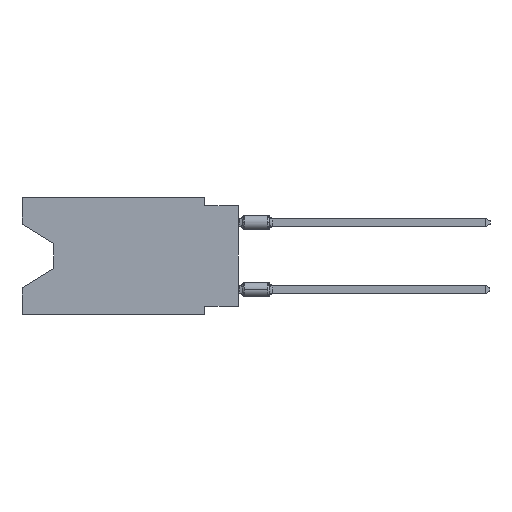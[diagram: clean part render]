
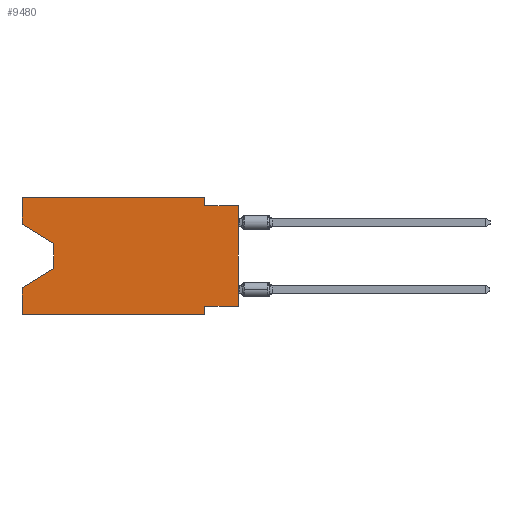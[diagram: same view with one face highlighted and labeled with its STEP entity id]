
A CAD part, left-side view. The second image highlights one B-rep face of the part: STEP entity #9480.
In plain terms, the highlighted planar face has unit normal (-1, 0, 0).
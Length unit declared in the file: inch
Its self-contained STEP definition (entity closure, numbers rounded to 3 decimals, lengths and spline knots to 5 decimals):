
#371 = VECTOR ( 'NONE', #15191, 39.37008 ) ;
#485 = ORIENTED_EDGE ( 'NONE', *, *, #4671, .T. ) ;
#795 = CARTESIAN_POINT ( 'NONE',  ( 0., 0.645, 0. ) ) ;
#812 = VECTOR ( 'NONE', #6958, 39.37008 ) ;
#1088 = DIRECTION ( 'NONE',  ( 0., 0., -1. ) ) ;
#1252 = EDGE_CURVE ( 'NONE', #9907, #4779, #9877, .T. ) ;
#1504 = CARTESIAN_POINT ( 'NONE',  ( 0., 0.1, 0. ) ) ;
#1529 = VECTOR ( 'NONE', #10505, 39.37008 ) ;
#1572 = CARTESIAN_POINT ( 'NONE',  ( 0., 0.55, -0.138 ) ) ;
#1799 = DIRECTION ( 'NONE',  ( 0., 0., -1. ) ) ;
#2082 = CARTESIAN_POINT ( 'NONE',  ( 0., 0.55, -0.138 ) ) ;
#2111 = EDGE_CURVE ( 'NONE', #5982, #10717, #15539, .T. ) ;
#2290 = LINE ( 'NONE', #8749, #15847 ) ;
#2360 = CARTESIAN_POINT ( 'NONE',  ( 0., 0.645, 0. ) ) ;
#2517 = ORIENTED_EDGE ( 'NONE', *, *, #13369, .T. ) ;
#2615 = DIRECTION ( 'NONE',  ( 0., 0.855, -0.519 ) ) ;
#2619 = CARTESIAN_POINT ( 'NONE',  ( 0., 0., -0.325 ) ) ;
#2694 = EDGE_CURVE ( 'NONE', #9907, #5982, #6921, .T. ) ;
#2731 = LINE ( 'NONE', #14497, #12615 ) ;
#3199 = LINE ( 'NONE', #2082, #11906 ) ;
#3293 = CARTESIAN_POINT ( 'NONE',  ( 0., 0., 0. ) ) ;
#4060 = CARTESIAN_POINT ( 'NONE',  ( 0., 0.645, -0.35 ) ) ;
#4140 = VECTOR ( 'NONE', #1088, 39.37008 ) ;
#4315 = CARTESIAN_POINT ( 'NONE',  ( 0., 0.645, 0. ) ) ;
#4490 = CARTESIAN_POINT ( 'NONE',  ( 0., 0., -0.025 ) ) ;
#4505 = LINE ( 'NONE', #10729, #12338 ) ;
#4671 = EDGE_CURVE ( 'NONE', #10297, #6731, #5054, .T. ) ;
#4779 = VERTEX_POINT ( 'NONE', #1572 ) ;
#5054 = LINE ( 'NONE', #6681, #1529 ) ;
#5093 = CARTESIAN_POINT ( 'NONE',  ( 0., 0.1, -0.325 ) ) ;
#5242 = VECTOR ( 'NONE', #8517, 39.37008 ) ;
#5277 = VECTOR ( 'NONE', #8826, 39.37008 ) ;
#5513 = LINE ( 'NONE', #13450, #812 ) ;
#5671 = EDGE_LOOP ( 'NONE', ( #11980, #5673, #2517, #9174, #485, #11666, #10380, #16726, #8176, #7142, #15026, #9383 ) ) ;
#5673 = ORIENTED_EDGE ( 'NONE', *, *, #7826, .T. ) ;
#5726 = VERTEX_POINT ( 'NONE', #13965 ) ;
#5751 = CARTESIAN_POINT ( 'NONE',  ( 0., 0.1, -0.025 ) ) ;
#5925 = DIRECTION ( 'NONE',  ( 0., 0., 1. ) ) ;
#5982 = VERTEX_POINT ( 'NONE', #4315 ) ;
#5990 = CARTESIAN_POINT ( 'NONE',  ( 0., 0., -0.025 ) ) ;
#6426 = PLANE ( 'NONE',  #16548 ) ;
#6441 = CARTESIAN_POINT ( 'NONE',  ( 0., 0.1, 0. ) ) ;
#6681 = CARTESIAN_POINT ( 'NONE',  ( 0., 0.645, -0.35 ) ) ;
#6731 = VERTEX_POINT ( 'NONE', #10371 ) ;
#6921 = LINE ( 'NONE', #795, #15919 ) ;
#6958 = DIRECTION ( 'NONE',  ( 0., 1., 0. ) ) ;
#7142 = ORIENTED_EDGE ( 'NONE', *, *, #13329, .F. ) ;
#7204 = VERTEX_POINT ( 'NONE', #2619 ) ;
#7277 = DIRECTION ( 'NONE',  ( 0., 0., -1. ) ) ;
#7405 = VECTOR ( 'NONE', #5925, 39.37008 ) ;
#7781 = DIRECTION ( 'NONE',  ( 0., 0., -1. ) ) ;
#7826 = EDGE_CURVE ( 'NONE', #4779, #8871, #3199, .T. ) ;
#7827 = VERTEX_POINT ( 'NONE', #5751 ) ;
#7869 = FACE_OUTER_BOUND ( 'NONE', #5671, .T. ) ;
#8176 = ORIENTED_EDGE ( 'NONE', *, *, #11539, .F. ) ;
#8517 = DIRECTION ( 'NONE',  ( 0., -0.855, -0.519 ) ) ;
#8749 = CARTESIAN_POINT ( 'NONE',  ( 0., 0.55, -0.212 ) ) ;
#8826 = DIRECTION ( 'NONE',  ( 0., -1., 0. ) ) ;
#8871 = VERTEX_POINT ( 'NONE', #12601 ) ;
#9174 = ORIENTED_EDGE ( 'NONE', *, *, #16521, .F. ) ;
#9248 = EDGE_CURVE ( 'NONE', #7204, #16286, #5513, .T. ) ;
#9383 = ORIENTED_EDGE ( 'NONE', *, *, #2694, .F. ) ;
#9480 = ADVANCED_FACE ( 'NONE', ( #7869 ), #6426, .F. ) ;
#9704 = CARTESIAN_POINT ( 'NONE',  ( 0., 0.645, -0.08025 ) ) ;
#9877 = LINE ( 'NONE', #9704, #5242 ) ;
#9907 = VERTEX_POINT ( 'NONE', #10642 ) ;
#10012 = EDGE_CURVE ( 'NONE', #16286, #6731, #4505, .T. ) ;
#10297 = VERTEX_POINT ( 'NONE', #4060 ) ;
#10371 = CARTESIAN_POINT ( 'NONE',  ( 0., 0.1, -0.35 ) ) ;
#10380 = ORIENTED_EDGE ( 'NONE', *, *, #9248, .F. ) ;
#10505 = DIRECTION ( 'NONE',  ( 0., -1., 0. ) ) ;
#10642 = CARTESIAN_POINT ( 'NONE',  ( 0., 0.645, -0.08025 ) ) ;
#10717 = VERTEX_POINT ( 'NONE', #1504 ) ;
#10729 = CARTESIAN_POINT ( 'NONE',  ( 0., 0.1, -0.35 ) ) ;
#11068 = LINE ( 'NONE', #6441, #4140 ) ;
#11119 = VERTEX_POINT ( 'NONE', #4490 ) ;
#11539 = EDGE_CURVE ( 'NONE', #7827, #11119, #12731, .T. ) ;
#11666 = ORIENTED_EDGE ( 'NONE', *, *, #10012, .F. ) ;
#11849 = DIRECTION ( 'NONE',  ( 0., 0., 1. ) ) ;
#11906 = VECTOR ( 'NONE', #7277, 39.37008 ) ;
#11980 = ORIENTED_EDGE ( 'NONE', *, *, #1252, .T. ) ;
#12338 = VECTOR ( 'NONE', #1799, 39.37008 ) ;
#12601 = CARTESIAN_POINT ( 'NONE',  ( 0., 0.55, -0.212 ) ) ;
#12615 = VECTOR ( 'NONE', #11849, 39.37008 ) ;
#12731 = LINE ( 'NONE', #5990, #371 ) ;
#12993 = CARTESIAN_POINT ( 'NONE',  ( 0., 0.645, 0. ) ) ;
#13329 = EDGE_CURVE ( 'NONE', #10717, #7827, #11068, .T. ) ;
#13369 = EDGE_CURVE ( 'NONE', #8871, #5726, #2290, .T. ) ;
#13450 = CARTESIAN_POINT ( 'NONE',  ( 0., 0., -0.325 ) ) ;
#13625 = EDGE_CURVE ( 'NONE', #7204, #11119, #14965, .T. ) ;
#13965 = CARTESIAN_POINT ( 'NONE',  ( 0., 0.645, -0.26975 ) ) ;
#14497 = CARTESIAN_POINT ( 'NONE',  ( 0., 0.645, 0. ) ) ;
#14767 = DIRECTION ( 'NONE',  ( 0., 0., 1. ) ) ;
#14965 = LINE ( 'NONE', #3293, #7405 ) ;
#15026 = ORIENTED_EDGE ( 'NONE', *, *, #2111, .F. ) ;
#15191 = DIRECTION ( 'NONE',  ( 0., -1., 0. ) ) ;
#15374 = DIRECTION ( 'NONE',  ( 1., 0., 0. ) ) ;
#15539 = LINE ( 'NONE', #2360, #5277 ) ;
#15847 = VECTOR ( 'NONE', #2615, 39.37008 ) ;
#15919 = VECTOR ( 'NONE', #14767, 39.37008 ) ;
#16286 = VERTEX_POINT ( 'NONE', #5093 ) ;
#16521 = EDGE_CURVE ( 'NONE', #10297, #5726, #2731, .T. ) ;
#16548 = AXIS2_PLACEMENT_3D ( 'NONE', #12993, #15374, #7781 ) ;
#16726 = ORIENTED_EDGE ( 'NONE', *, *, #13625, .T. ) ;
